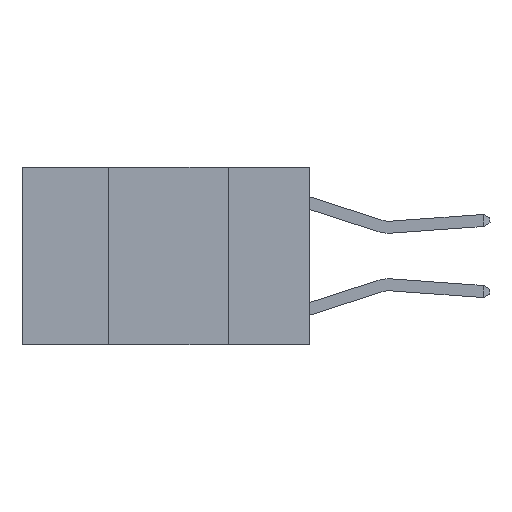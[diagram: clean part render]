
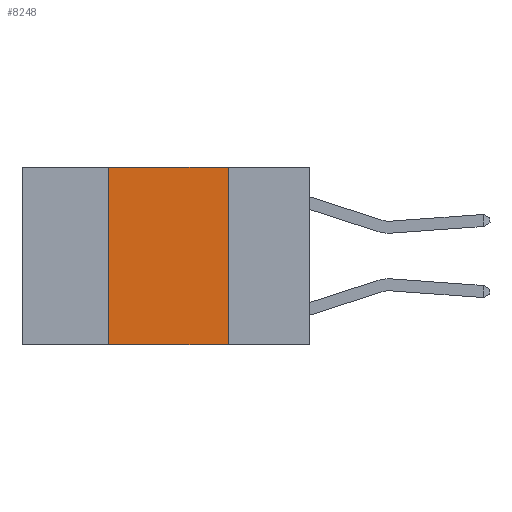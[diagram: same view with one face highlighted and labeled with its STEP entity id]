
A CAD part, left-side view. The second image highlights one B-rep face of the part: STEP entity #8248.
In plain terms, the highlighted planar face has unit normal (-1, 0, 0).
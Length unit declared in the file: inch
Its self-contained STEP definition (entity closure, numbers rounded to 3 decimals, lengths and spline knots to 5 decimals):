
#701 = CARTESIAN_POINT ( 'NONE',  ( 0., 0.6, 0. ) ) ;
#2021 = ORIENTED_EDGE ( 'NONE', *, *, #17383, .F. ) ;
#3081 = DIRECTION ( 'NONE',  ( 0., 0., -1. ) ) ;
#3522 = ORIENTED_EDGE ( 'NONE', *, *, #18950, .F. ) ;
#6578 = VERTEX_POINT ( 'NONE', #23555 ) ;
#7697 = EDGE_CURVE ( 'NONE', #26795, #6578, #8884, .T. ) ;
#8248 = ADVANCED_FACE ( 'NONE', ( #18418 ), #26519, .F. ) ;
#8884 = LINE ( 'NONE', #15204, #26836 ) ;
#10771 = CARTESIAN_POINT ( 'NONE',  ( 0., 0.42, -0.37 ) ) ;
#12445 = AXIS2_PLACEMENT_3D ( 'NONE', #701, #17237, #3081 ) ;
#12828 = DIRECTION ( 'NONE',  ( 0., -1., 0. ) ) ;
#13585 = DIRECTION ( 'NONE',  ( 0., 0., -1. ) ) ;
#14394 = LINE ( 'NONE', #29916, #26829 ) ;
#15204 = CARTESIAN_POINT ( 'NONE',  ( 0., 0.6, 0. ) ) ;
#16078 = ORIENTED_EDGE ( 'NONE', *, *, #22086, .T. ) ;
#16512 = VERTEX_POINT ( 'NONE', #22237 ) ;
#17237 = DIRECTION ( 'NONE',  ( 1., 0., 0. ) ) ;
#17383 = EDGE_CURVE ( 'NONE', #6578, #16512, #14394, .T. ) ;
#17962 = VECTOR ( 'NONE', #24069, 39.37008 ) ;
#18418 = FACE_OUTER_BOUND ( 'NONE', #21466, .T. ) ;
#18950 = EDGE_CURVE ( 'NONE', #21305, #26795, #24163, .T. ) ;
#21305 = VERTEX_POINT ( 'NONE', #10771 ) ;
#21466 = EDGE_LOOP ( 'NONE', ( #2021, #27760, #3522, #16078 ) ) ;
#21726 = CARTESIAN_POINT ( 'NONE',  ( 0., 0.42, 0. ) ) ;
#22086 = EDGE_CURVE ( 'NONE', #21305, #16512, #27599, .T. ) ;
#22237 = CARTESIAN_POINT ( 'NONE',  ( 0., 0.17, -0.37 ) ) ;
#22965 = DIRECTION ( 'NONE',  ( 0., -1., 0. ) ) ;
#23555 = CARTESIAN_POINT ( 'NONE',  ( 0., 0.17, 0. ) ) ;
#24069 = DIRECTION ( 'NONE',  ( 0., 0., 1. ) ) ;
#24163 = LINE ( 'NONE', #21726, #17962 ) ;
#25303 = CARTESIAN_POINT ( 'NONE',  ( 0., 0.6, -0.37 ) ) ;
#26519 = PLANE ( 'NONE',  #12445 ) ;
#26795 = VERTEX_POINT ( 'NONE', #30392 ) ;
#26829 = VECTOR ( 'NONE', #13585, 39.37008 ) ;
#26836 = VECTOR ( 'NONE', #12828, 39.37008 ) ;
#26876 = VECTOR ( 'NONE', #22965, 39.37008 ) ;
#27599 = LINE ( 'NONE', #25303, #26876 ) ;
#27760 = ORIENTED_EDGE ( 'NONE', *, *, #7697, .F. ) ;
#29916 = CARTESIAN_POINT ( 'NONE',  ( 0., 0.17, 0. ) ) ;
#30392 = CARTESIAN_POINT ( 'NONE',  ( 0., 0.42, 0. ) ) ;
